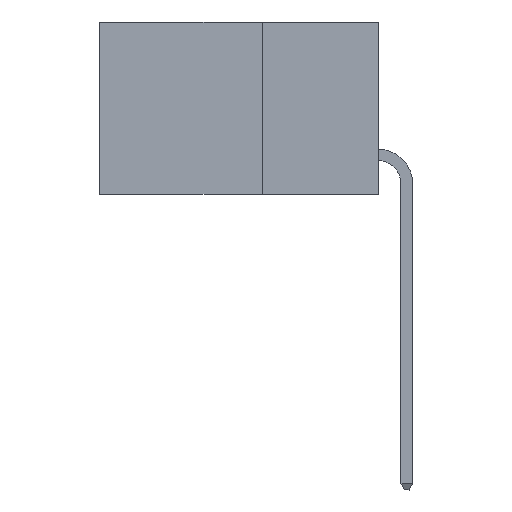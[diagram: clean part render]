
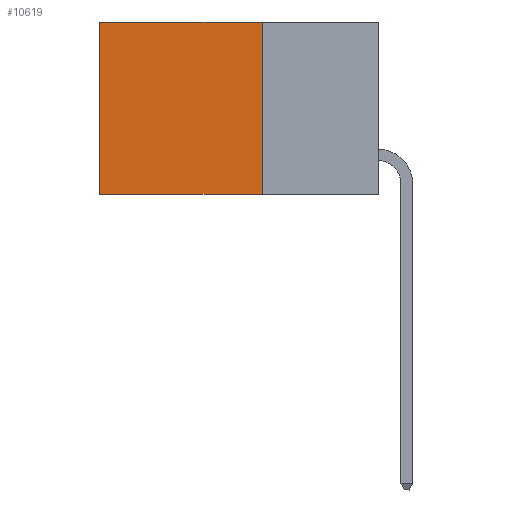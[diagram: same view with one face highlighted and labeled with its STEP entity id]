
A CAD part, left-side view. The second image highlights one B-rep face of the part: STEP entity #10619.
In plain terms, the highlighted planar face has unit normal (-1, 0, 0).
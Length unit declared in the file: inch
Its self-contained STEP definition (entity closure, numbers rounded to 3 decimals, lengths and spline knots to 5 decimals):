
#102 = DIRECTION ( 'NONE',  ( 0., 1., 0. ) ) ;
#148 = VECTOR ( 'NONE', #12977, 39.37008 ) ;
#169 = LINE ( 'NONE', #327, #12267 ) ;
#221 = ORIENTED_EDGE ( 'NONE', *, *, #5826, .T. ) ;
#265 = VECTOR ( 'NONE', #722, 39.37008 ) ;
#327 = CARTESIAN_POINT ( 'NONE',  ( 0.298, 0.25, -0.37 ) ) ;
#722 = DIRECTION ( 'NONE',  ( 0., 0., -1. ) ) ;
#1081 = CARTESIAN_POINT ( 'NONE',  ( 0.298, 0.25, 0. ) ) ;
#2337 = EDGE_CURVE ( 'NONE', #4858, #14640, #7402, .T. ) ;
#2817 = ORIENTED_EDGE ( 'NONE', *, *, #9642, .F. ) ;
#2925 = FACE_OUTER_BOUND ( 'NONE', #15316, .T. ) ;
#3980 = VERTEX_POINT ( 'NONE', #14275 ) ;
#4054 = CARTESIAN_POINT ( 'NONE',  ( 0.298, 0.25, 0. ) ) ;
#4858 = VERTEX_POINT ( 'NONE', #4054 ) ;
#5826 = EDGE_CURVE ( 'NONE', #4858, #10693, #9014, .T. ) ;
#6158 = EDGE_CURVE ( 'NONE', #10693, #3980, #10523, .T. ) ;
#7181 = DIRECTION ( 'NONE',  ( 0., 0., -1. ) ) ;
#7271 = VECTOR ( 'NONE', #7181, 39.37008 ) ;
#7402 = LINE ( 'NONE', #1081, #265 ) ;
#7449 = CARTESIAN_POINT ( 'NONE',  ( 0.298, 0.6, 0. ) ) ;
#7538 = ORIENTED_EDGE ( 'NONE', *, *, #6158, .T. ) ;
#9014 = LINE ( 'NONE', #13237, #148 ) ;
#9458 = ORIENTED_EDGE ( 'NONE', *, *, #2337, .F. ) ;
#9642 = EDGE_CURVE ( 'NONE', #14640, #3980, #169, .T. ) ;
#9989 = AXIS2_PLACEMENT_3D ( 'NONE', #13993, #13979, #13958 ) ;
#10149 = CARTESIAN_POINT ( 'NONE',  ( 0.298, 0.25, -0.37 ) ) ;
#10523 = LINE ( 'NONE', #7449, #7271 ) ;
#10619 = ADVANCED_FACE ( 'NONE', ( #2925 ), #14026, .F. ) ;
#10693 = VERTEX_POINT ( 'NONE', #13488 ) ;
#12267 = VECTOR ( 'NONE', #102, 39.37008 ) ;
#12977 = DIRECTION ( 'NONE',  ( 0., 1., 0. ) ) ;
#13237 = CARTESIAN_POINT ( 'NONE',  ( 0.298, 0.25, 0. ) ) ;
#13488 = CARTESIAN_POINT ( 'NONE',  ( 0.298, 0.6, 0. ) ) ;
#13958 = DIRECTION ( 'NONE',  ( 0., 0., -1. ) ) ;
#13979 = DIRECTION ( 'NONE',  ( 1., 0., 0. ) ) ;
#13993 = CARTESIAN_POINT ( 'NONE',  ( 0.298, 0.25, 0. ) ) ;
#14026 = PLANE ( 'NONE',  #9989 ) ;
#14275 = CARTESIAN_POINT ( 'NONE',  ( 0.298, 0.6, -0.37 ) ) ;
#14640 = VERTEX_POINT ( 'NONE', #10149 ) ;
#15316 = EDGE_LOOP ( 'NONE', ( #7538, #2817, #9458, #221 ) ) ;
